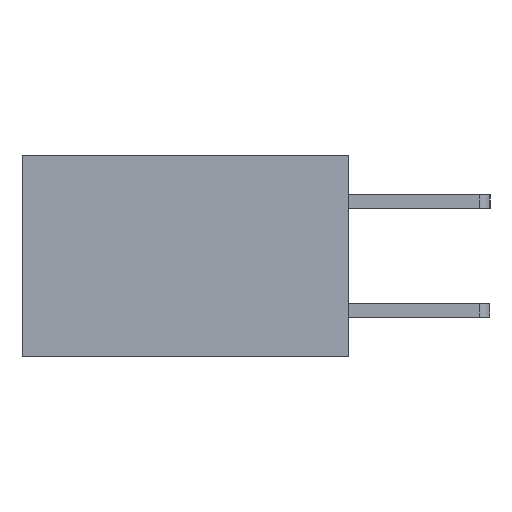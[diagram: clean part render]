
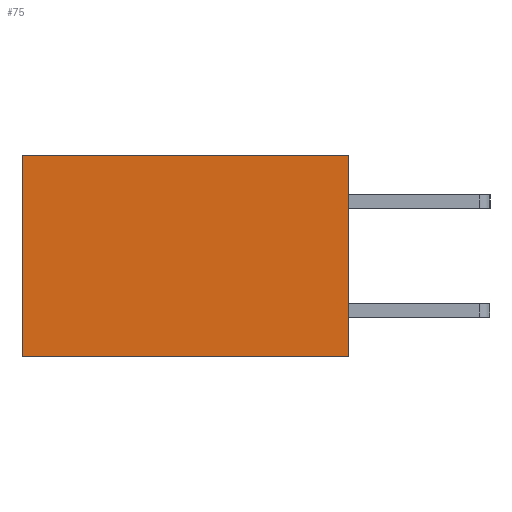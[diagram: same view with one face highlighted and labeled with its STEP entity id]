
A CAD part, left-side view. The second image highlights one B-rep face of the part: STEP entity #75.
In plain terms, the highlighted planar face has unit normal (-1, 0, 0).
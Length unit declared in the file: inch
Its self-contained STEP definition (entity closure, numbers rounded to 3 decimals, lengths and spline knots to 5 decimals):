
#43 = LINE ( 'NONE', #6119, #11723 ) ;
#75 = ADVANCED_FACE ( 'NONE', ( #7945 ), #3483, .F. ) ;
#243 = VERTEX_POINT ( 'NONE', #255 ) ;
#255 = CARTESIAN_POINT ( 'NONE',  ( 0.298, 0.6, 0. ) ) ;
#553 = ORIENTED_EDGE ( 'NONE', *, *, #3574, .T. ) ;
#1782 = CARTESIAN_POINT ( 'NONE',  ( 0.298, 0., -0.37 ) ) ;
#2043 = VERTEX_POINT ( 'NONE', #7551 ) ;
#2896 = VECTOR ( 'NONE', #10788, 39.37008 ) ;
#3178 = DIRECTION ( 'NONE',  ( 1., 0., 0. ) ) ;
#3218 = ORIENTED_EDGE ( 'NONE', *, *, #6374, .T. ) ;
#3483 = PLANE ( 'NONE',  #6966 ) ;
#3574 = EDGE_CURVE ( 'NONE', #243, #7564, #9605, .T. ) ;
#4651 = CARTESIAN_POINT ( 'NONE',  ( 0.298, 0., 0. ) ) ;
#4996 = DIRECTION ( 'NONE',  ( 0., 0., -1. ) ) ;
#5439 = LINE ( 'NONE', #6369, #2896 ) ;
#5771 = DIRECTION ( 'NONE',  ( 0., 1., 0. ) ) ;
#6119 = CARTESIAN_POINT ( 'NONE',  ( 0.298, 0., 0. ) ) ;
#6369 = CARTESIAN_POINT ( 'NONE',  ( 0.298, 0., -0.37 ) ) ;
#6374 = EDGE_CURVE ( 'NONE', #2043, #243, #43, .T. ) ;
#6499 = VECTOR ( 'NONE', #10047, 39.37008 ) ;
#6786 = CARTESIAN_POINT ( 'NONE',  ( 0.298, 0.6, 0. ) ) ;
#6929 = EDGE_CURVE ( 'NONE', #8817, #7564, #5439, .T. ) ;
#6966 = AXIS2_PLACEMENT_3D ( 'NONE', #4651, #3178, #7067 ) ;
#7067 = DIRECTION ( 'NONE',  ( 0., 0., -1. ) ) ;
#7184 = VECTOR ( 'NONE', #4996, 39.37008 ) ;
#7506 = EDGE_CURVE ( 'NONE', #2043, #8817, #8963, .T. ) ;
#7551 = CARTESIAN_POINT ( 'NONE',  ( 0.298, 0., 0. ) ) ;
#7564 = VERTEX_POINT ( 'NONE', #9591 ) ;
#7655 = ORIENTED_EDGE ( 'NONE', *, *, #6929, .F. ) ;
#7945 = FACE_OUTER_BOUND ( 'NONE', #9426, .T. ) ;
#8348 = ORIENTED_EDGE ( 'NONE', *, *, #7506, .F. ) ;
#8817 = VERTEX_POINT ( 'NONE', #1782 ) ;
#8963 = LINE ( 'NONE', #10072, #6499 ) ;
#9426 = EDGE_LOOP ( 'NONE', ( #553, #7655, #8348, #3218 ) ) ;
#9591 = CARTESIAN_POINT ( 'NONE',  ( 0.298, 0.6, -0.37 ) ) ;
#9605 = LINE ( 'NONE', #6786, #7184 ) ;
#10047 = DIRECTION ( 'NONE',  ( 0., 0., -1. ) ) ;
#10072 = CARTESIAN_POINT ( 'NONE',  ( 0.298, 0., 0. ) ) ;
#10788 = DIRECTION ( 'NONE',  ( 0., 1., 0. ) ) ;
#11723 = VECTOR ( 'NONE', #5771, 39.37008 ) ;
